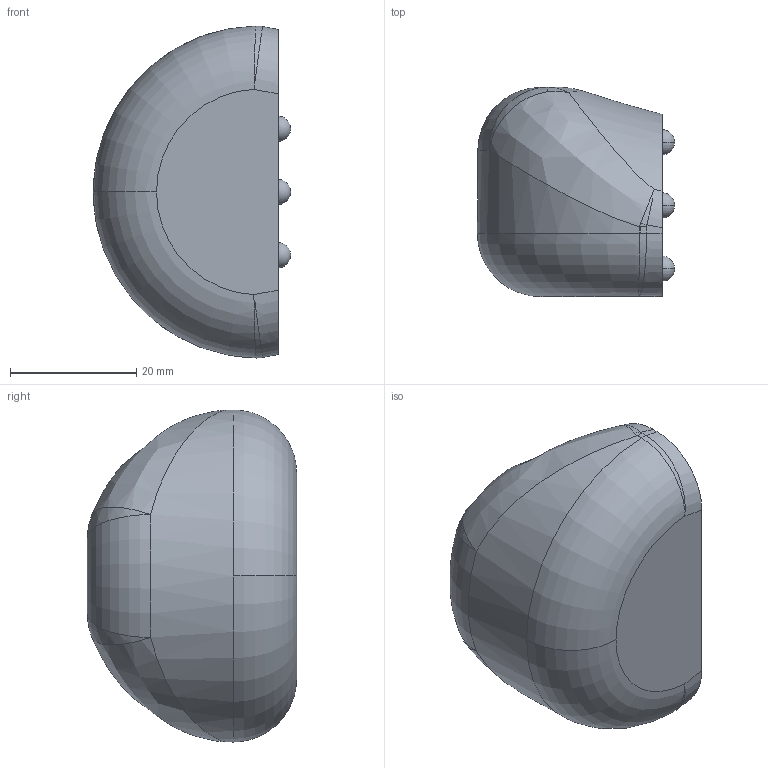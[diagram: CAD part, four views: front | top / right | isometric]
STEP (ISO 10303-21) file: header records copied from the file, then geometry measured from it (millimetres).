
FILE_DESCRIPTION (( 'STEP AP214' ), '1' );
FILE_NAME ('Stock Knob.STEP', '2013-06-24T22:49:40', ( 'Asher' ), ( '' ), 'SwSTEP 2.0', 'SolidWorks 2013', '' );
FILE_SCHEMA (( 'AUTOMOTIVE_DESIGN' ));
Length unit declared in the file: millimetre
Products named in the file (1): Stock Knob
Bounding box: 31.23 x 33.09 x 52.53 mm (x, y, z)
Volume: 32914 mm3; surface area: 5585.9 mm2
Topology: 1 solids, 1 shells, 40 faces, 102 edges, 56 vertices
Faces by surface type: sphere 12, bspline 11, torus 7, cylinder 7, plane 3
Entity records: 1788 total; most frequent: CARTESIAN_POINT 971, ORIENTED_EDGE 164, DIRECTION 161, EDGE_CURVE 82, AXIS2_PLACEMENT_3D 76, VERTEX_POINT 48, CIRCLE 46, EDGE_LOOP 44
